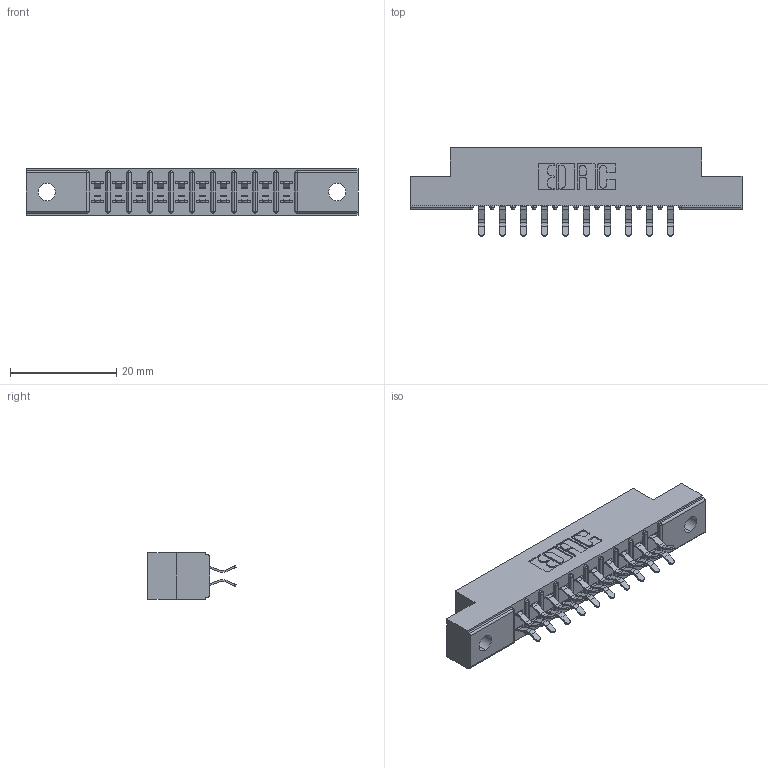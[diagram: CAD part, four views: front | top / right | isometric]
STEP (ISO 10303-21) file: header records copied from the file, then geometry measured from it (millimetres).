
FILE_DESCRIPTION (( 'STEP AP203' ), '1' );
FILE_NAME ('355-020-556-202.STEP', '2019-09-11T03:38:23', ( '' ), ( '' ), 'SwSTEP 2.0', 'SolidWorks 2016', '' );
FILE_SCHEMA (( 'CONFIG_CONTROL_DESIGN' ));
Length unit declared in the file: inch
Products named in the file (3): 355-020-556-202; 305 Part_.128 Dia; 305-290-001_556
Assembly tree (21 placements, depth 2):
  355-020-556-202
    305 Part_.128 Dia
    305-290-001_556  x20
Bounding box: 62.64 x 16.64 x 8.71 mm (x, y, z)
Volume: 3903 mm3; surface area: 6431.7 mm2
Topology: 21 solids, 21 shells, 1236 faces, 3546 edges, 2308 vertices
Faces by surface type: plane 688, cylinder 508, sphere 40
Entity records: 14947 total; most frequent: CARTESIAN_POINT 2476, ORIENTED_EDGE 2452, DIRECTION 2424, EDGE_CURVE 1226, VECTOR 952, LINE 952, VERTEX_POINT 788, AXIS2_PLACEMENT_3D 736
